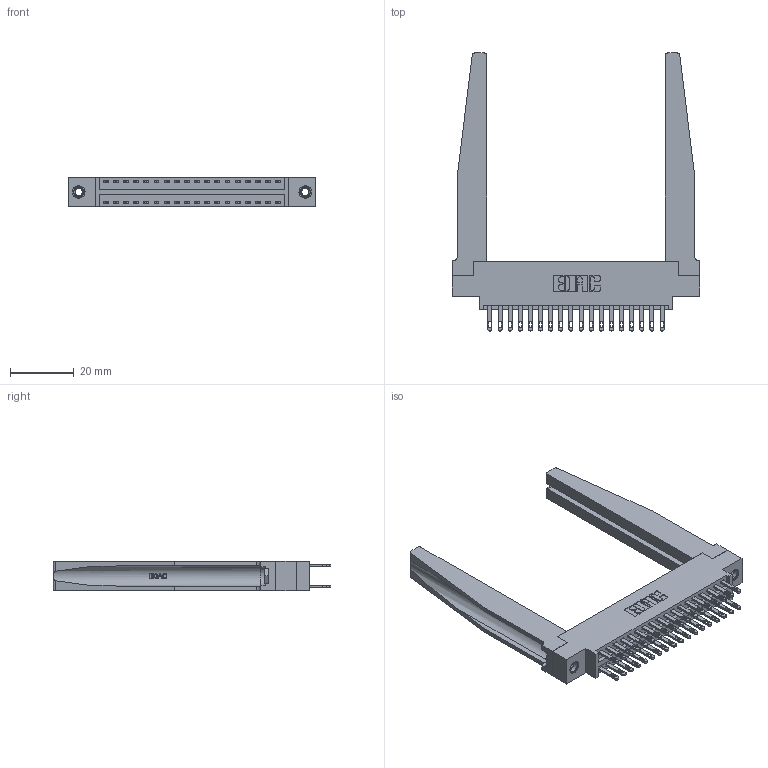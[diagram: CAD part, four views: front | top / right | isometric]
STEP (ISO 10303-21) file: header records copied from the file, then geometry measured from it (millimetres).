
FILE_DESCRIPTION (( 'STEP AP203' ), '1' );
FILE_NAME ('346-036-500-878.STEP', '2022-05-19T20:54:41', ( '' ), ( '' ), 'SwSTEP 2.0', 'SolidWorks 2020', '' );
FILE_SCHEMA (( 'CONFIG_CONTROL_DESIGN' ));
Length unit declared in the file: inch
Products named in the file (5): 346-036-500-878; 346 Part_0.170 Offset - 0.156 Dia-TH; 345-250-001_345-250-001-102; 345-292-001_345-293-100; 346-220-078_345-220-078
Assembly tree (41 placements, depth 2):
  346-036-500-878
    346 Part_0.170 Offset - 0.156 Dia-TH
    345-292-001_345-293-100  x36
    346-220-078_345-220-078  x2
    345-250-001_345-250-001-102  x2
Bounding box: 77.72 x 87.12 x 9.4 mm (x, y, z)
Volume: 14238.8 mm3; surface area: 16826.8 mm2
Topology: 41 solids, 41 shells, 2102 faces, 6277 edges, 4174 vertices
Faces by surface type: plane 1280, cylinder 770, bspline 36, cone 12, torus 4
Entity records: 20204 total; most frequent: CARTESIAN_POINT 4305, ORIENTED_EDGE 3126, DIRECTION 2833, EDGE_CURVE 1563, VECTOR 1261, LINE 1261, VERTEX_POINT 1036, AXIS2_PLACEMENT_3D 786
